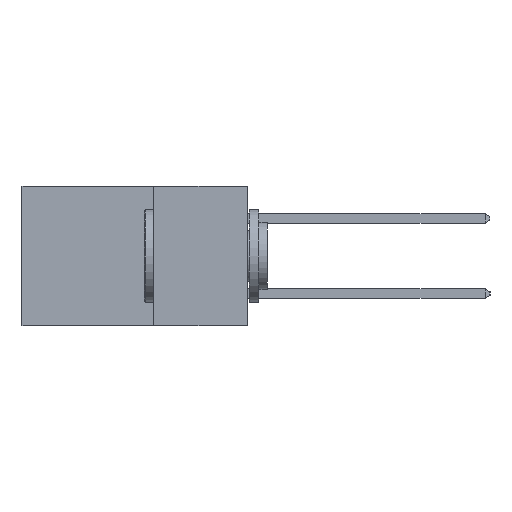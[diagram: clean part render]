
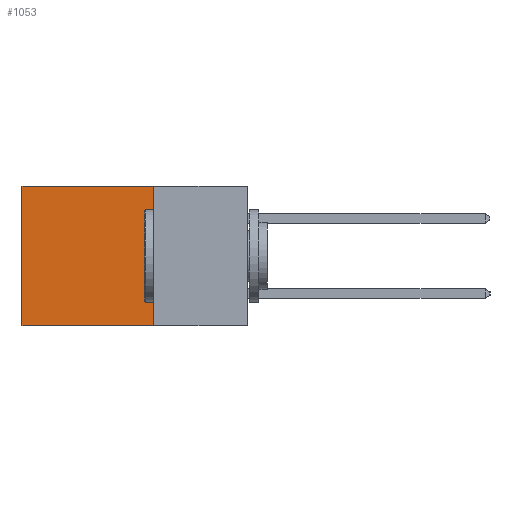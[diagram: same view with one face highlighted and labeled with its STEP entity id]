
A CAD part, left-side view. The second image highlights one B-rep face of the part: STEP entity #1053.
In plain terms, the highlighted planar face has unit normal (-1, 0, 0).
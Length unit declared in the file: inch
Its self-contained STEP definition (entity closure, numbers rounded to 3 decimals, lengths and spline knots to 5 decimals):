
#197 = EDGE_CURVE ( 'NONE', #5220, #18489, #22721, .T. ) ;
#262 = CARTESIAN_POINT ( 'NONE',  ( 0.2615, 0.6, -0.37 ) ) ;
#1053 = ADVANCED_FACE ( 'NONE', ( #17596 ), #18675, .F. ) ;
#2147 = CARTESIAN_POINT ( 'NONE',  ( 0.2615, 0.25, 0. ) ) ;
#2661 = ORIENTED_EDGE ( 'NONE', *, *, #197, .F. ) ;
#3460 = CARTESIAN_POINT ( 'NONE',  ( 0.2615, 0.25, -0.37 ) ) ;
#4110 = DIRECTION ( 'NONE',  ( 0., 1., 0. ) ) ;
#4496 = DIRECTION ( 'NONE',  ( 0., 1., 0. ) ) ;
#5220 = VERTEX_POINT ( 'NONE', #12882 ) ;
#5284 = ORIENTED_EDGE ( 'NONE', *, *, #22437, .F. ) ;
#6600 = VECTOR ( 'NONE', #11077, 39.37008 ) ;
#7331 = VECTOR ( 'NONE', #16152, 39.37008 ) ;
#7550 = AXIS2_PLACEMENT_3D ( 'NONE', #17759, #19126, #19076 ) ;
#7704 = VERTEX_POINT ( 'NONE', #262 ) ;
#9035 = ORIENTED_EDGE ( 'NONE', *, *, #20373, .T. ) ;
#9910 = VECTOR ( 'NONE', #4496, 39.37008 ) ;
#10037 = EDGE_LOOP ( 'NONE', ( #20698, #5284, #2661, #9035 ) ) ;
#10421 = EDGE_CURVE ( 'NONE', #22907, #7704, #17713, .T. ) ;
#11077 = DIRECTION ( 'NONE',  ( 0., 0., -1. ) ) ;
#11172 = LINE ( 'NONE', #14393, #9910 ) ;
#11591 = LINE ( 'NONE', #2147, #21179 ) ;
#11849 = CARTESIAN_POINT ( 'NONE',  ( 0.2615, 0.6, 0. ) ) ;
#12882 = CARTESIAN_POINT ( 'NONE',  ( 0.2615, 0.25, 0. ) ) ;
#14393 = CARTESIAN_POINT ( 'NONE',  ( 0.2615, 0.25, -0.37 ) ) ;
#15977 = CARTESIAN_POINT ( 'NONE',  ( 0.2615, 0.6, -0.37 ) ) ;
#16152 = DIRECTION ( 'NONE',  ( 0., 0., -1. ) ) ;
#17596 = FACE_OUTER_BOUND ( 'NONE', #10037, .T. ) ;
#17713 = LINE ( 'NONE', #15977, #7331 ) ;
#17759 = CARTESIAN_POINT ( 'NONE',  ( 0.2615, 0.25, -0.37 ) ) ;
#18489 = VERTEX_POINT ( 'NONE', #3460 ) ;
#18675 = PLANE ( 'NONE',  #7550 ) ;
#19076 = DIRECTION ( 'NONE',  ( 0., 0., -1. ) ) ;
#19126 = DIRECTION ( 'NONE',  ( 1., 0., 0. ) ) ;
#20373 = EDGE_CURVE ( 'NONE', #5220, #22907, #11591, .T. ) ;
#20698 = ORIENTED_EDGE ( 'NONE', *, *, #10421, .T. ) ;
#21179 = VECTOR ( 'NONE', #4110, 39.37008 ) ;
#22437 = EDGE_CURVE ( 'NONE', #18489, #7704, #11172, .T. ) ;
#22721 = LINE ( 'NONE', #24499, #6600 ) ;
#22907 = VERTEX_POINT ( 'NONE', #11849 ) ;
#24499 = CARTESIAN_POINT ( 'NONE',  ( 0.2615, 0.25, -0.37 ) ) ;
